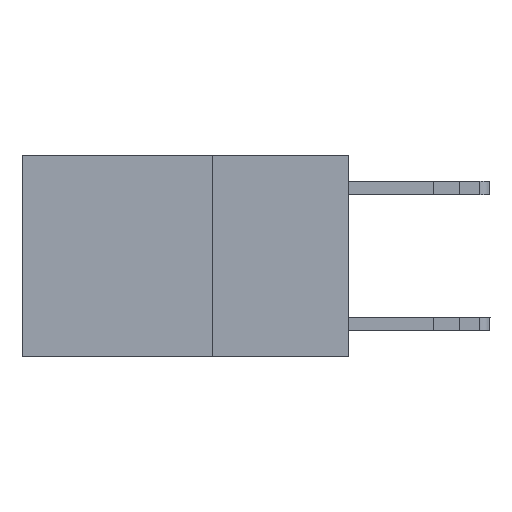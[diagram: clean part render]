
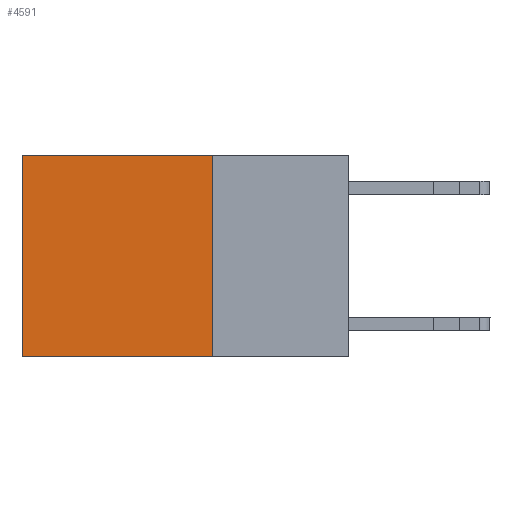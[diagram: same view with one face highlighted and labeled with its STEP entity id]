
A CAD part, left-side view. The second image highlights one B-rep face of the part: STEP entity #4591.
In plain terms, the highlighted planar face has unit normal (-1, 0, 0).
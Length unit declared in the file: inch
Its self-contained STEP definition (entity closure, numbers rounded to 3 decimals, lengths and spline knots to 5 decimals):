
#186 = EDGE_CURVE ( 'NONE', #15149, #16400, #19877, .T. ) ;
#935 = DIRECTION ( 'NONE',  ( 0., 0., -1. ) ) ;
#1073 = DIRECTION ( 'NONE',  ( 1., 0., 0. ) ) ;
#1163 = CARTESIAN_POINT ( 'NONE',  ( 0.2625, 0.25, 0. ) ) ;
#1691 = PLANE ( 'NONE',  #21286 ) ;
#2479 = LINE ( 'NONE', #21100, #2582 ) ;
#2582 = VECTOR ( 'NONE', #20574, 39.37008 ) ;
#3501 = DIRECTION ( 'NONE',  ( 0., 1., 0. ) ) ;
#3555 = CARTESIAN_POINT ( 'NONE',  ( 0.2625, 0.25, 0. ) ) ;
#3558 = VERTEX_POINT ( 'NONE', #15068 ) ;
#4011 = CARTESIAN_POINT ( 'NONE',  ( 0.2625, 0.25, -0.37 ) ) ;
#4591 = ADVANCED_FACE ( 'NONE', ( #17722 ), #1691, .F. ) ;
#7074 = DIRECTION ( 'NONE',  ( 0., 0., -1. ) ) ;
#7159 = CARTESIAN_POINT ( 'NONE',  ( 0.2625, 0.6, 0. ) ) ;
#7485 = ORIENTED_EDGE ( 'NONE', *, *, #11317, .T. ) ;
#9046 = CARTESIAN_POINT ( 'NONE',  ( 0.2625, 0.25, 0. ) ) ;
#9811 = ORIENTED_EDGE ( 'NONE', *, *, #186, .T. ) ;
#10026 = EDGE_LOOP ( 'NONE', ( #7485, #19685, #20266, #9811 ) ) ;
#10244 = CARTESIAN_POINT ( 'NONE',  ( 0.2625, 0.25, -0.37 ) ) ;
#11317 = EDGE_CURVE ( 'NONE', #16400, #3558, #18698, .T. ) ;
#14002 = LINE ( 'NONE', #10244, #14224 ) ;
#14224 = VECTOR ( 'NONE', #21950, 39.37008 ) ;
#15068 = CARTESIAN_POINT ( 'NONE',  ( 0.2625, 0.6, -0.37 ) ) ;
#15149 = VERTEX_POINT ( 'NONE', #9046 ) ;
#16400 = VERTEX_POINT ( 'NONE', #18657 ) ;
#17643 = EDGE_CURVE ( 'NONE', #15149, #19748, #2479, .T. ) ;
#17722 = FACE_OUTER_BOUND ( 'NONE', #10026, .T. ) ;
#18657 = CARTESIAN_POINT ( 'NONE',  ( 0.2625, 0.6, 0. ) ) ;
#18692 = VECTOR ( 'NONE', #7074, 39.37008 ) ;
#18698 = LINE ( 'NONE', #7159, #18692 ) ;
#19685 = ORIENTED_EDGE ( 'NONE', *, *, #21863, .F. ) ;
#19748 = VERTEX_POINT ( 'NONE', #4011 ) ;
#19877 = LINE ( 'NONE', #3555, #20222 ) ;
#20222 = VECTOR ( 'NONE', #3501, 39.37008 ) ;
#20266 = ORIENTED_EDGE ( 'NONE', *, *, #17643, .F. ) ;
#20574 = DIRECTION ( 'NONE',  ( 0., 0., -1. ) ) ;
#21100 = CARTESIAN_POINT ( 'NONE',  ( 0.2625, 0.25, 0. ) ) ;
#21286 = AXIS2_PLACEMENT_3D ( 'NONE', #1163, #1073, #935 ) ;
#21863 = EDGE_CURVE ( 'NONE', #19748, #3558, #14002, .T. ) ;
#21950 = DIRECTION ( 'NONE',  ( 0., 1., 0. ) ) ;
